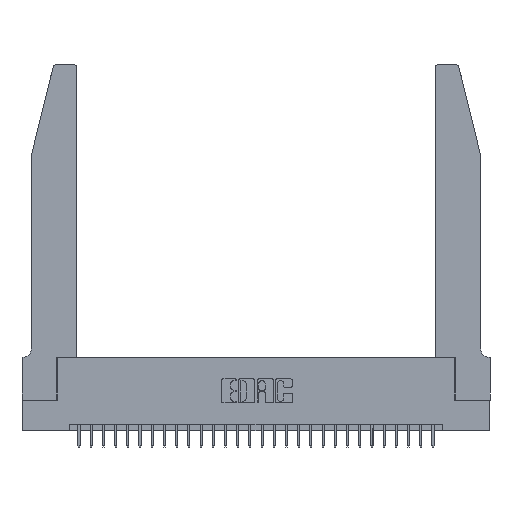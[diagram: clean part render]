
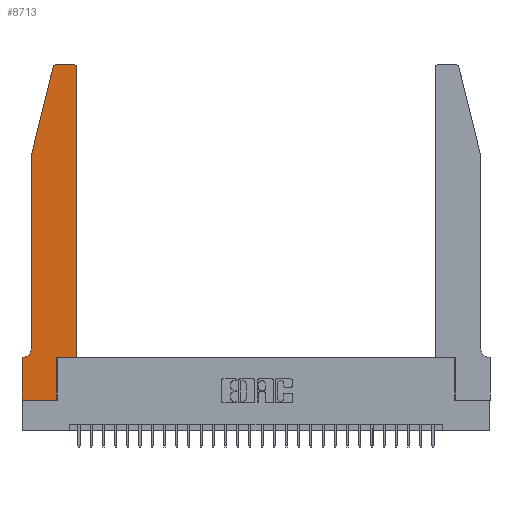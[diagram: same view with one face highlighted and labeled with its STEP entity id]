
A CAD part, top view. The second image highlights one B-rep face of the part: STEP entity #8713.
In plain terms, the highlighted planar face has unit normal (0, 0, 1).
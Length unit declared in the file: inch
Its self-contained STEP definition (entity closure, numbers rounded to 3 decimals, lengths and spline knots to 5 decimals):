
#710 = DIRECTION ( 'NONE',  ( 0., 1., 0. ) ) ;
#1157 = LINE ( 'NONE', #19718, #25501 ) ;
#2253 = CARTESIAN_POINT ( 'NONE',  ( 0.4505, 2.72, 0.37 ) ) ;
#2578 = EDGE_CURVE ( 'NONE', #7841, #12105, #27344, .T. ) ;
#2628 = CARTESIAN_POINT ( 'NONE',  ( 0.2865, 0., 0.37 ) ) ;
#2746 = VERTEX_POINT ( 'NONE', #17583 ) ;
#2776 = EDGE_CURVE ( 'NONE', #2746, #25399, #6470, .T. ) ;
#3065 = EDGE_CURVE ( 'NONE', #25399, #19537, #14413, .T. ) ;
#3415 = DIRECTION ( 'NONE',  ( -1., 0., 0. ) ) ;
#3462 = EDGE_CURVE ( 'NONE', #20199, #2746, #5264, .T. ) ;
#4596 = ORIENTED_EDGE ( 'NONE', *, *, #6853, .T. ) ;
#4824 = LINE ( 'NONE', #16521, #18784 ) ;
#5264 = LINE ( 'NONE', #26660, #12497 ) ;
#5918 = VECTOR ( 'NONE', #10863, 39.37008 ) ;
#6470 = LINE ( 'NONE', #18495, #13466 ) ;
#6853 = EDGE_CURVE ( 'NONE', #9737, #7841, #12991, .T. ) ;
#7319 = AXIS2_PLACEMENT_3D ( 'NONE', #24560, #29408, #29113 ) ;
#7841 = VERTEX_POINT ( 'NONE', #14508 ) ;
#8142 = ORIENTED_EDGE ( 'NONE', *, *, #26545, .T. ) ;
#8144 = LINE ( 'NONE', #19885, #5918 ) ;
#8243 = CARTESIAN_POINT ( 'NONE',  ( 0.0055, 0.42, 0.37 ) ) ;
#8285 = AXIS2_PLACEMENT_3D ( 'NONE', #24707, #13124, #10690 ) ;
#8453 = AXIS2_PLACEMENT_3D ( 'NONE', #17938, #13363, #15479 ) ;
#8489 = VERTEX_POINT ( 'NONE', #18369 ) ;
#8712 = EDGE_CURVE ( 'NONE', #14393, #14753, #19479, .T. ) ;
#8713 = ADVANCED_FACE ( 'NONE', ( #26810 ), #18023, .T. ) ;
#9211 = ORIENTED_EDGE ( 'NONE', *, *, #15714, .T. ) ;
#9359 = CARTESIAN_POINT ( 'NONE',  ( 0.0055, 0.35, 0.37 ) ) ;
#9579 = AXIS2_PLACEMENT_3D ( 'NONE', #8243, #27099, #3415 ) ;
#9737 = VERTEX_POINT ( 'NONE', #25341 ) ;
#10423 = EDGE_CURVE ( 'NONE', #26046, #14393, #17211, .T. ) ;
#10690 = DIRECTION ( 'NONE',  ( 1., 0., 0. ) ) ;
#10863 = DIRECTION ( 'NONE',  ( 1., 0., 0. ) ) ;
#11020 = ORIENTED_EDGE ( 'NONE', *, *, #3065, .T. ) ;
#11215 = DIRECTION ( 'NONE',  ( 1., 0., 0. ) ) ;
#11950 = EDGE_CURVE ( 'NONE', #12508, #26046, #8144, .T. ) ;
#12105 = VERTEX_POINT ( 'NONE', #2628 ) ;
#12497 = VECTOR ( 'NONE', #21834, 39.37008 ) ;
#12508 = VERTEX_POINT ( 'NONE', #23029 ) ;
#12991 = LINE ( 'NONE', #22004, #15001 ) ;
#13124 = DIRECTION ( 'NONE',  ( 0., 0., 1. ) ) ;
#13143 = VECTOR ( 'NONE', #11215, 39.37008 ) ;
#13363 = DIRECTION ( 'NONE',  ( 0., 0., 1. ) ) ;
#13466 = VECTOR ( 'NONE', #15734, 39.37008 ) ;
#14393 = VERTEX_POINT ( 'NONE', #2253 ) ;
#14403 = CARTESIAN_POINT ( 'NONE',  ( 0.4505, 0.35, 0.37 ) ) ;
#14413 = CIRCLE ( 'NONE', #9579, 0.07 ) ;
#14508 = CARTESIAN_POINT ( 'NONE',  ( 0., 0., 0.37 ) ) ;
#14753 = VERTEX_POINT ( 'NONE', #17880 ) ;
#15001 = VECTOR ( 'NONE', #22292, 39.37008 ) ;
#15230 = EDGE_CURVE ( 'NONE', #14753, #8489, #25583, .T. ) ;
#15479 = DIRECTION ( 'NONE',  ( 1., 0., 0. ) ) ;
#15714 = EDGE_CURVE ( 'NONE', #8489, #20199, #23092, .T. ) ;
#15734 = DIRECTION ( 'NONE',  ( 0., -1., 0. ) ) ;
#16161 = CARTESIAN_POINT ( 'NONE',  ( 0.2605, 2.75, 0.37 ) ) ;
#16521 = CARTESIAN_POINT ( 'NONE',  ( 0.0755, 0.35, 0.37 ) ) ;
#16554 = VECTOR ( 'NONE', #26610, 39.37008 ) ;
#17211 = LINE ( 'NONE', #19658, #16554 ) ;
#17512 = EDGE_LOOP ( 'NONE', ( #26877, #9211, #25729, #22823, #11020, #29768, #4596, #24919, #8142, #27329, #20635, #27374 ) ) ;
#17583 = CARTESIAN_POINT ( 'NONE',  ( 0.0755, 2., 0.37 ) ) ;
#17880 = CARTESIAN_POINT ( 'NONE',  ( 0.4205, 2.75, 0.37 ) ) ;
#17938 = CARTESIAN_POINT ( 'NONE',  ( 0.284, 2.72, 0.37 ) ) ;
#18023 = PLANE ( 'NONE',  #8285 ) ;
#18369 = CARTESIAN_POINT ( 'NONE',  ( 0.284, 2.75, 0.37 ) ) ;
#18495 = CARTESIAN_POINT ( 'NONE',  ( 0.0755, 2., 0.37 ) ) ;
#18784 = VECTOR ( 'NONE', #23818, 39.37008 ) ;
#19479 = CIRCLE ( 'NONE', #7319, 0.03 ) ;
#19537 = VERTEX_POINT ( 'NONE', #9359 ) ;
#19658 = CARTESIAN_POINT ( 'NONE',  ( 0.4505, 0.35, 0.37 ) ) ;
#19675 = VECTOR ( 'NONE', #25444, 39.37008 ) ;
#19718 = CARTESIAN_POINT ( 'NONE',  ( 0.2865, 0.35, 0.37 ) ) ;
#19885 = CARTESIAN_POINT ( 'NONE',  ( 0.4505, 0.35, 0.37 ) ) ;
#20199 = VERTEX_POINT ( 'NONE', #29509 ) ;
#20635 = ORIENTED_EDGE ( 'NONE', *, *, #10423, .T. ) ;
#21834 = DIRECTION ( 'NONE',  ( -0.239, -0.971, 0. ) ) ;
#22004 = CARTESIAN_POINT ( 'NONE',  ( 0., 0., 0.37 ) ) ;
#22292 = DIRECTION ( 'NONE',  ( 0., -1., 0. ) ) ;
#22823 = ORIENTED_EDGE ( 'NONE', *, *, #2776, .T. ) ;
#22968 = CARTESIAN_POINT ( 'NONE',  ( 0., 0., 0.37 ) ) ;
#23029 = CARTESIAN_POINT ( 'NONE',  ( 0.2865, 0.35, 0.37 ) ) ;
#23092 = CIRCLE ( 'NONE', #8453, 0.03 ) ;
#23818 = DIRECTION ( 'NONE',  ( -1., 0., 0. ) ) ;
#24560 = CARTESIAN_POINT ( 'NONE',  ( 0.4205, 2.72, 0.37 ) ) ;
#24707 = CARTESIAN_POINT ( 'NONE',  ( 0., 0.35, 0.37 ) ) ;
#24919 = ORIENTED_EDGE ( 'NONE', *, *, #2578, .T. ) ;
#25341 = CARTESIAN_POINT ( 'NONE',  ( 0., 0.35, 0.37 ) ) ;
#25399 = VERTEX_POINT ( 'NONE', #27825 ) ;
#25444 = DIRECTION ( 'NONE',  ( -1., 0., 0. ) ) ;
#25501 = VECTOR ( 'NONE', #710, 39.37008 ) ;
#25583 = LINE ( 'NONE', #16161, #19675 ) ;
#25729 = ORIENTED_EDGE ( 'NONE', *, *, #3462, .T. ) ;
#26046 = VERTEX_POINT ( 'NONE', #14403 ) ;
#26545 = EDGE_CURVE ( 'NONE', #12105, #12508, #1157, .T. ) ;
#26610 = DIRECTION ( 'NONE',  ( 0., 1., 0. ) ) ;
#26660 = CARTESIAN_POINT ( 'NONE',  ( 0.0755, 2., 0.37 ) ) ;
#26810 = FACE_OUTER_BOUND ( 'NONE', #17512, .T. ) ;
#26877 = ORIENTED_EDGE ( 'NONE', *, *, #15230, .T. ) ;
#27099 = DIRECTION ( 'NONE',  ( 0., 0., -1. ) ) ;
#27329 = ORIENTED_EDGE ( 'NONE', *, *, #11950, .T. ) ;
#27344 = LINE ( 'NONE', #22968, #13143 ) ;
#27374 = ORIENTED_EDGE ( 'NONE', *, *, #8712, .T. ) ;
#27825 = CARTESIAN_POINT ( 'NONE',  ( 0.0755, 0.42, 0.37 ) ) ;
#27844 = EDGE_CURVE ( 'NONE', #19537, #9737, #4824, .T. ) ;
#29113 = DIRECTION ( 'NONE',  ( 1., 0., 0. ) ) ;
#29408 = DIRECTION ( 'NONE',  ( 0., 0., 1. ) ) ;
#29509 = CARTESIAN_POINT ( 'NONE',  ( 0.25487, 2.72718, 0.37 ) ) ;
#29768 = ORIENTED_EDGE ( 'NONE', *, *, #27844, .T. ) ;
